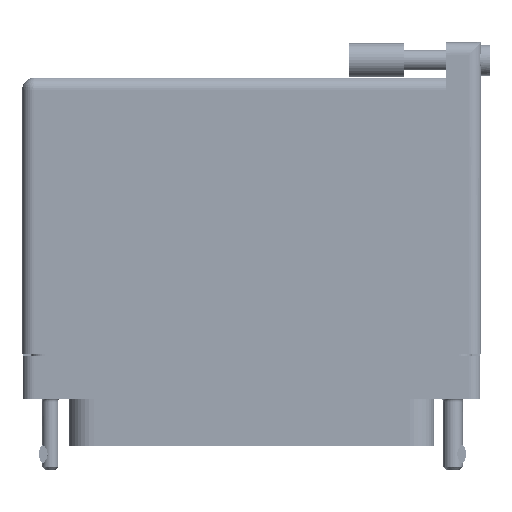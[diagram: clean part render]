
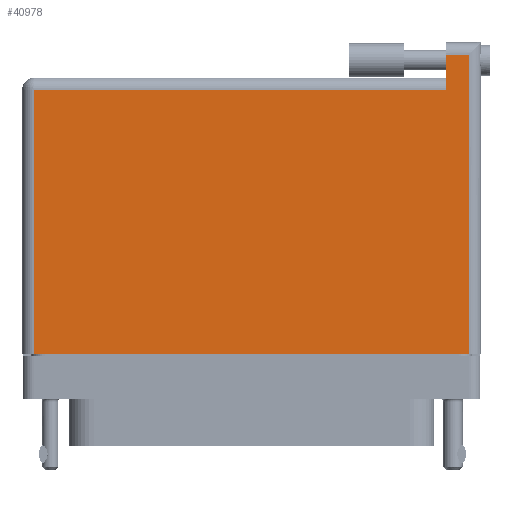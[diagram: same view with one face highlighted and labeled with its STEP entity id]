
A CAD part, front view. The second image highlights one B-rep face of the part: STEP entity #40978.
In plain terms, the highlighted face is planar.
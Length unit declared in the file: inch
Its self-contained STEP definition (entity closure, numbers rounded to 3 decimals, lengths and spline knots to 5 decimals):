
#135 = CARTESIAN_POINT ( 'NONE',  ( -1.23, -0.1, 0.4495 ) ) ;
#236 = CARTESIAN_POINT ( 'NONE',  ( -1.23, -0.1, 0.4495 ) ) ;
#3425 = CARTESIAN_POINT ( 'NONE',  ( -1.23, 1.396, 0.4495 ) ) ;
#3486 = VERTEX_POINT ( 'NONE', #49526 ) ;
#4143 = CARTESIAN_POINT ( 'NONE',  ( 1.103, 1.596, 0.4495 ) ) ;
#6170 = DIRECTION ( 'NONE',  ( 0., 0., -1. ) ) ;
#6442 = AXIS2_PLACEMENT_3D ( 'NONE', #34541, #6170, #39319 ) ;
#6902 = CARTESIAN_POINT ( 'NONE',  ( 1.23, -0.1, 0.4495 ) ) ;
#7227 = LINE ( 'NONE', #40677, #21897 ) ;
#7303 = EDGE_CURVE ( 'NONE', #42528, #9925, #38533, .T. ) ;
#7693 = ORIENTED_EDGE ( 'NONE', *, *, #35757, .T. ) ;
#7798 = VECTOR ( 'NONE', #54963, 39.37008 ) ;
#8318 = LINE ( 'NONE', #135, #13426 ) ;
#9925 = VERTEX_POINT ( 'NONE', #6902 ) ;
#13426 = VECTOR ( 'NONE', #52082, 39.37008 ) ;
#14216 = VECTOR ( 'NONE', #55086, 39.37008 ) ;
#14281 = EDGE_CURVE ( 'NONE', #55809, #42528, #8318, .T. ) ;
#17124 = LINE ( 'NONE', #49401, #19349 ) ;
#19349 = VECTOR ( 'NONE', #40519, 39.37008 ) ;
#20831 = LINE ( 'NONE', #26017, #14216 ) ;
#21732 = DIRECTION ( 'NONE',  ( 0., -1., 0. ) ) ;
#21897 = VECTOR ( 'NONE', #21732, 39.37008 ) ;
#23635 = ORIENTED_EDGE ( 'NONE', *, *, #14281, .T. ) ;
#23780 = VECTOR ( 'NONE', #55703, 39.37008 ) ;
#24247 = EDGE_LOOP ( 'NONE', ( #37384, #37267, #44261, #7693, #58560, #23635 ) ) ;
#24855 = PLANE ( 'NONE',  #6442 ) ;
#26017 = CARTESIAN_POINT ( 'NONE',  ( -1.3, 1.596, 0.4495 ) ) ;
#26531 = EDGE_CURVE ( 'NONE', #9925, #37739, #17124, .T. ) ;
#30108 = VERTEX_POINT ( 'NONE', #4143 ) ;
#31834 = CARTESIAN_POINT ( 'NONE',  ( -1.3, -0.1, 0.4495 ) ) ;
#32776 = LINE ( 'NONE', #40733, #7798 ) ;
#34541 = CARTESIAN_POINT ( 'NONE',  ( -1.3, 1.466, 0.4495 ) ) ;
#35757 = EDGE_CURVE ( 'NONE', #30108, #3486, #7227, .T. ) ;
#35831 = FACE_OUTER_BOUND ( 'NONE', #24247, .T. ) ;
#37267 = ORIENTED_EDGE ( 'NONE', *, *, #26531, .T. ) ;
#37384 = ORIENTED_EDGE ( 'NONE', *, *, #7303, .T. ) ;
#37739 = VERTEX_POINT ( 'NONE', #53156 ) ;
#38533 = LINE ( 'NONE', #31834, #23780 ) ;
#39319 = DIRECTION ( 'NONE',  ( -1., 0., 0. ) ) ;
#40519 = DIRECTION ( 'NONE',  ( 0., 1., 0. ) ) ;
#40677 = CARTESIAN_POINT ( 'NONE',  ( 1.103, 1.666, 0.4495 ) ) ;
#40733 = CARTESIAN_POINT ( 'NONE',  ( -1.3, 1.396, 0.4495 ) ) ;
#40978 = ADVANCED_FACE ( 'NONE', ( #35831 ), #24855, .F. ) ;
#42528 = VERTEX_POINT ( 'NONE', #236 ) ;
#44261 = ORIENTED_EDGE ( 'NONE', *, *, #59469, .T. ) ;
#49401 = CARTESIAN_POINT ( 'NONE',  ( 1.23, 1.666, 0.4495 ) ) ;
#49526 = CARTESIAN_POINT ( 'NONE',  ( 1.103, 1.396, 0.4495 ) ) ;
#50925 = EDGE_CURVE ( 'NONE', #3486, #55809, #32776, .T. ) ;
#52082 = DIRECTION ( 'NONE',  ( 0., -1., 0. ) ) ;
#53156 = CARTESIAN_POINT ( 'NONE',  ( 1.23, 1.596, 0.4495 ) ) ;
#54963 = DIRECTION ( 'NONE',  ( -1., 0., 0. ) ) ;
#55086 = DIRECTION ( 'NONE',  ( -1., 0., 0. ) ) ;
#55703 = DIRECTION ( 'NONE',  ( 1., 0., 0. ) ) ;
#55809 = VERTEX_POINT ( 'NONE', #3425 ) ;
#58560 = ORIENTED_EDGE ( 'NONE', *, *, #50925, .T. ) ;
#59469 = EDGE_CURVE ( 'NONE', #37739, #30108, #20831, .T. ) ;
